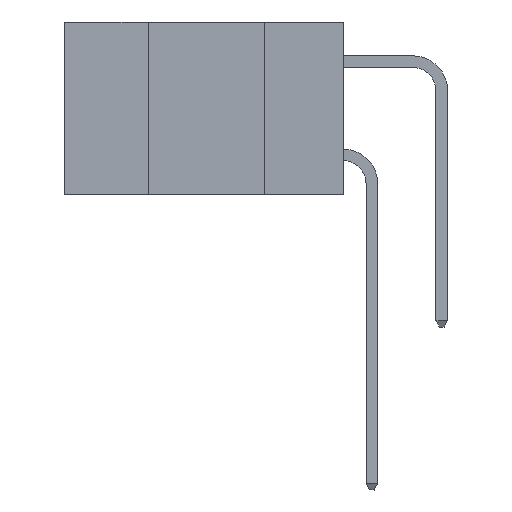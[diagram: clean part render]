
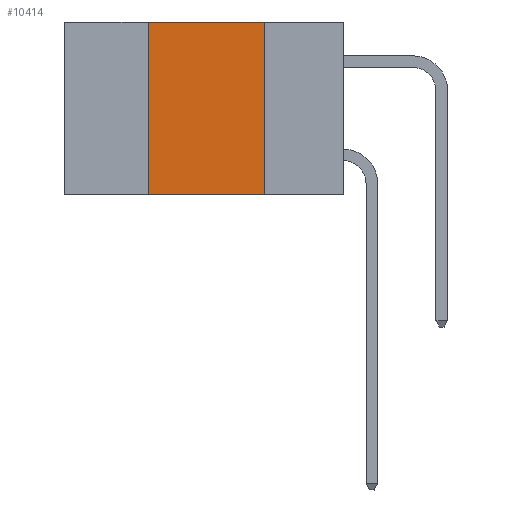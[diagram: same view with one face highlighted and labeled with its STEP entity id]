
A CAD part, left-side view. The second image highlights one B-rep face of the part: STEP entity #10414.
In plain terms, the highlighted planar face has unit normal (-1, 0, 0).
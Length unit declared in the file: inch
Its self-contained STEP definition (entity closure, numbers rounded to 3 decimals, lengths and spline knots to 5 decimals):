
#111 = EDGE_CURVE ( 'NONE', #2627, #9279, #4535, .T. ) ;
#360 = ORIENTED_EDGE ( 'NONE', *, *, #1658, .F. ) ;
#495 = CARTESIAN_POINT ( 'NONE',  ( 0., 0.17, 0. ) ) ;
#727 = EDGE_CURVE ( 'NONE', #2627, #11283, #8519, .T. ) ;
#733 = CARTESIAN_POINT ( 'NONE',  ( 0., 0.6, -0.37 ) ) ;
#1599 = VECTOR ( 'NONE', #4088, 39.37008 ) ;
#1653 = ORIENTED_EDGE ( 'NONE', *, *, #111, .F. ) ;
#1658 = EDGE_CURVE ( 'NONE', #9279, #14552, #4160, .T. ) ;
#1693 = DIRECTION ( 'NONE',  ( 0., 0., -1. ) ) ;
#1977 = PLANE ( 'NONE',  #8402 ) ;
#2573 = CARTESIAN_POINT ( 'NONE',  ( 0., 0.17, -0.37 ) ) ;
#2627 = VERTEX_POINT ( 'NONE', #7962 ) ;
#3000 = FACE_OUTER_BOUND ( 'NONE', #8428, .T. ) ;
#3352 = CARTESIAN_POINT ( 'NONE',  ( 0., 0.42, 0. ) ) ;
#4088 = DIRECTION ( 'NONE',  ( 0., -1., 0. ) ) ;
#4160 = LINE ( 'NONE', #9565, #1599 ) ;
#4535 = LINE ( 'NONE', #5960, #9440 ) ;
#4759 = DIRECTION ( 'NONE',  ( 0., 0., 1. ) ) ;
#5356 = CARTESIAN_POINT ( 'NONE',  ( 0., 0.17, -0.37 ) ) ;
#5960 = CARTESIAN_POINT ( 'NONE',  ( 0., 0.42, -0.37 ) ) ;
#6318 = VECTOR ( 'NONE', #7079, 39.37008 ) ;
#7079 = DIRECTION ( 'NONE',  ( 0., 0., -1. ) ) ;
#7587 = DIRECTION ( 'NONE',  ( 1., 0., 0. ) ) ;
#7962 = CARTESIAN_POINT ( 'NONE',  ( 0., 0.42, -0.37 ) ) ;
#8270 = ORIENTED_EDGE ( 'NONE', *, *, #11125, .F. ) ;
#8402 = AXIS2_PLACEMENT_3D ( 'NONE', #13200, #7587, #1693 ) ;
#8428 = EDGE_LOOP ( 'NONE', ( #8270, #360, #1653, #8982 ) ) ;
#8519 = LINE ( 'NONE', #733, #11583 ) ;
#8982 = ORIENTED_EDGE ( 'NONE', *, *, #727, .T. ) ;
#9279 = VERTEX_POINT ( 'NONE', #3352 ) ;
#9440 = VECTOR ( 'NONE', #4759, 39.37008 ) ;
#9565 = CARTESIAN_POINT ( 'NONE',  ( 0., 0.6, 0. ) ) ;
#10414 = ADVANCED_FACE ( 'NONE', ( #3000 ), #1977, .F. ) ;
#11125 = EDGE_CURVE ( 'NONE', #14552, #11283, #12678, .T. ) ;
#11283 = VERTEX_POINT ( 'NONE', #5356 ) ;
#11583 = VECTOR ( 'NONE', #13040, 39.37008 ) ;
#12678 = LINE ( 'NONE', #2573, #6318 ) ;
#13040 = DIRECTION ( 'NONE',  ( 0., -1., 0. ) ) ;
#13200 = CARTESIAN_POINT ( 'NONE',  ( 0., 0.6, 0. ) ) ;
#14552 = VERTEX_POINT ( 'NONE', #495 ) ;
